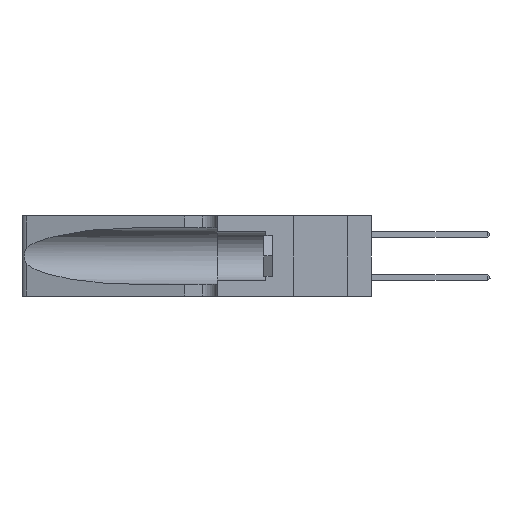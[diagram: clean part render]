
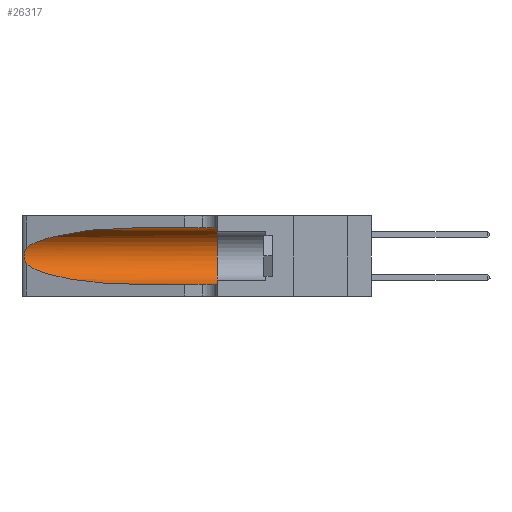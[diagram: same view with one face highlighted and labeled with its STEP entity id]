
A CAD part, left-side view. The second image highlights one B-rep face of the part: STEP entity #26317.
In plain terms, the highlighted cylindrical face has radius 3.308 mm (diameter 6.617 mm), a partial arc.
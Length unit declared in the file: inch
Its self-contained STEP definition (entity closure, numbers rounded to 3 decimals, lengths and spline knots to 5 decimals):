
#1200 = CARTESIAN_POINT ( 'NONE',  ( 0.25639, 1.23184, 0.21858 ) ) ;
#3497 = LINE ( 'NONE', #22711, #18288 ) ;
#5120 = CARTESIAN_POINT ( 'NONE',  ( 0.1305, 1.61858, 0.31525 ) ) ;
#5274 = CARTESIAN_POINT ( 'NONE',  ( 0.25487, 1.22718, 0.14631 ) ) ;
#6284 = EDGE_LOOP ( 'NONE', ( #17965, #6518, #35735, #36256, #22331, #18622 ) ) ;
#6518 = ORIENTED_EDGE ( 'NONE', *, *, #8142, .T. ) ;
#7354 = LINE ( 'NONE', #5120, #30026 ) ;
#7357 = VERTEX_POINT ( 'NONE', #32547 ) ;
#8008 = CARTESIAN_POINT ( 'NONE',  ( 0.25787, 1.23484, 0.2124 ) ) ;
#8142 = EDGE_CURVE ( 'NONE', #7357, #8435, #31179, .T. ) ;
#8243 = CARTESIAN_POINT ( 'NONE',  ( 0.25487, 1.22718, 0.22369 ) ) ;
#8435 = VERTEX_POINT ( 'NONE', #40047 ) ;
#8537 = CARTESIAN_POINT ( 'NONE',  ( 0.1305, 0.72297, 0.31525 ) ) ;
#9614 = DIRECTION ( 'NONE',  ( 0., 1., 0. ) ) ;
#9811 = AXIS2_PLACEMENT_3D ( 'NONE', #29779, #9614, #36863 ) ;
#11076 = EDGE_CURVE ( 'NONE', #34568, #39966, #7354, .T. ) ;
#11078 = EDGE_CURVE ( 'NONE', #34568, #7357, #40075, .T. ) ;
#11353 = CARTESIAN_POINT ( 'NONE',  ( 0.25487, 1.22718, 0.14631 ) ) ;
#11652 = CARTESIAN_POINT ( 'NONE',  ( 0.26075, 1.23896, 0.19203 ) ) ;
#12017 = CARTESIAN_POINT ( 'NONE',  ( 0.1305, 0.72297, 0.05475 ) ) ;
#13237 = VERTEX_POINT ( 'NONE', #27050 ) ;
#13543 = CARTESIAN_POINT ( 'NONE',  ( 0.25639, 1.23186, 0.15144 ) ) ;
#14441 = CARTESIAN_POINT ( 'NONE',  ( 0.25555, 1.22993, 0.14849 ) ) ;
#15354 = CARTESIAN_POINT ( 'NONE',  ( 0.25856, 1.23593, 0.16098 ) ) ;
#16508 = CARTESIAN_POINT ( 'NONE',  ( 0.25789, 1.23486, 0.15765 ) ) ;
#17853 = CARTESIAN_POINT ( 'NONE',  ( 0.25555, 1.22994, 0.2215 ) ) ;
#17965 = ORIENTED_EDGE ( 'NONE', *, *, #11078, .T. ) ;
#18021 = EDGE_CURVE ( 'NONE', #20091, #13237, #3497, .T. ) ;
#18207 = EDGE_CURVE ( 'NONE', #39966, #13237, #29850, .T. ) ;
#18232 = CARTESIAN_POINT ( 'NONE',  ( 0.18966, 0.96281, 0.31525 ) ) ;
#18288 = VECTOR ( 'NONE', #18925, 39.37008 ) ;
#18622 = ORIENTED_EDGE ( 'NONE', *, *, #11076, .F. ) ;
#18925 = DIRECTION ( 'NONE',  ( 0., -1., 0. ) ) ;
#19127 = EDGE_CURVE ( 'NONE', #8435, #20091, #22256, .T. ) ;
#19471 = CARTESIAN_POINT ( 'NONE',  ( 0.26017, 1.23833, 0.17102 ) ) ;
#19485 = AXIS2_PLACEMENT_3D ( 'NONE', #35336, #25994, #22201 ) ;
#20091 = VERTEX_POINT ( 'NONE', #12017 ) ;
#21274 = CARTESIAN_POINT ( 'NONE',  ( 0.1305, 0.72297, 0.31525 ) ) ;
#22201 = DIRECTION ( 'NONE',  ( 0., 0., -1. ) ) ;
#22256 =( BOUNDED_CURVE ( )  B_SPLINE_CURVE ( 3, ( #11353, #28341, #35255, #32276 ),
 .UNSPECIFIED., .F., .T. ) 
 B_SPLINE_CURVE_WITH_KNOTS ( ( 4, 4 ),
 ( 3.44316, 4.71239 ),
 .UNSPECIFIED. ) 
 CURVE ( )  GEOMETRIC_REPRESENTATION_ITEM ( )  RATIONAL_B_SPLINE_CURVE ( ( 1., 0.87, 0.87, 1. ) ) 
 REPRESENTATION_ITEM ( '' )  );
#22331 = ORIENTED_EDGE ( 'NONE', *, *, #18207, .F. ) ;
#22711 = CARTESIAN_POINT ( 'NONE',  ( 0.1305, 1.61858, 0.05475 ) ) ;
#25994 = DIRECTION ( 'NONE',  ( 0., -1., 0. ) ) ;
#26317 = ADVANCED_FACE ( 'NONE', ( #36795 ), #32579, .F. ) ;
#27050 = CARTESIAN_POINT ( 'NONE',  ( 0.1305, 0.35, 0.05475 ) ) ;
#28341 = CARTESIAN_POINT ( 'NONE',  ( 0.2373, 1.15595, 0.08982 ) ) ;
#28581 = CARTESIAN_POINT ( 'NONE',  ( 0.2373, 1.15595, 0.28018 ) ) ;
#29779 = CARTESIAN_POINT ( 'NONE',  ( 0.1305, 0.35, 0.185 ) ) ;
#29850 = CIRCLE ( 'NONE', #9811, 0.13025 ) ;
#30026 = VECTOR ( 'NONE', #31669, 39.37008 ) ;
#31179 = B_SPLINE_CURVE_WITH_KNOTS ( 'NONE', 3,
 ( #34677, #17853, #1200, #8008, #35111, #38480, #11652, #42093, #19471, #15354, #16508, #13543, #14441, #5274 ),
 .UNSPECIFIED., .F., .F.,
 ( 4, 2, 2, 2, 2, 2, 4 ),
 ( 0., 0.00027, 0.00053, 0.00107, 0.0016, 0.00187, 0.00214 ),
 .UNSPECIFIED. ) ;
#31669 = DIRECTION ( 'NONE',  ( 0., -1., 0. ) ) ;
#32276 = CARTESIAN_POINT ( 'NONE',  ( 0.1305, 0.72297, 0.05475 ) ) ;
#32547 = CARTESIAN_POINT ( 'NONE',  ( 0.25487, 1.22718, 0.22369 ) ) ;
#32579 = CYLINDRICAL_SURFACE ( 'NONE', #19485, 0.13025 ) ;
#34029 = CARTESIAN_POINT ( 'NONE',  ( 0.1305, 0.35, 0.31525 ) ) ;
#34568 = VERTEX_POINT ( 'NONE', #21274 ) ;
#34677 = CARTESIAN_POINT ( 'NONE',  ( 0.25487, 1.22718, 0.22369 ) ) ;
#35111 = CARTESIAN_POINT ( 'NONE',  ( 0.25854, 1.2359, 0.20912 ) ) ;
#35255 = CARTESIAN_POINT ( 'NONE',  ( 0.18966, 0.96281, 0.05475 ) ) ;
#35336 = CARTESIAN_POINT ( 'NONE',  ( 0.1305, 1.61858, 0.185 ) ) ;
#35735 = ORIENTED_EDGE ( 'NONE', *, *, #19127, .T. ) ;
#36256 = ORIENTED_EDGE ( 'NONE', *, *, #18021, .T. ) ;
#36795 = FACE_OUTER_BOUND ( 'NONE', #6284, .T. ) ;
#36863 = DIRECTION ( 'NONE',  ( 0., 0., 1. ) ) ;
#38480 = CARTESIAN_POINT ( 'NONE',  ( 0.26018, 1.23835, 0.19895 ) ) ;
#39966 = VERTEX_POINT ( 'NONE', #34029 ) ;
#40047 = CARTESIAN_POINT ( 'NONE',  ( 0.25487, 1.22718, 0.14631 ) ) ;
#40075 =( BOUNDED_CURVE ( )  B_SPLINE_CURVE ( 3, ( #8537, #18232, #28581, #8243 ),
 .UNSPECIFIED., .F., .F. ) 
 B_SPLINE_CURVE_WITH_KNOTS ( ( 4, 4 ),
 ( 1.5708, 2.84003 ),
 .UNSPECIFIED. ) 
 CURVE ( )  GEOMETRIC_REPRESENTATION_ITEM ( )  RATIONAL_B_SPLINE_CURVE ( ( 1., 0.87, 0.87, 1. ) ) 
 REPRESENTATION_ITEM ( '' )  );
#42093 = CARTESIAN_POINT ( 'NONE',  ( 0.26075, 1.23896, 0.178 ) ) ;
